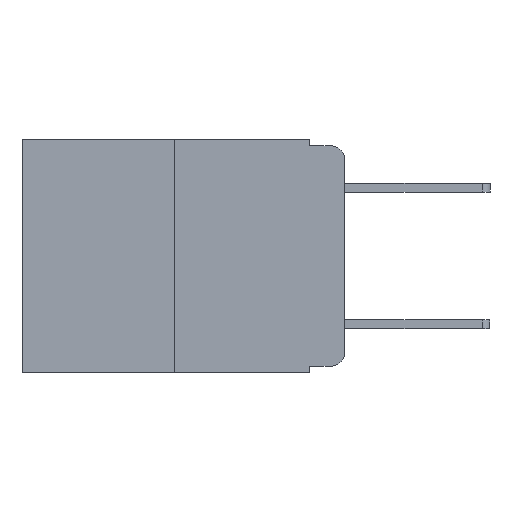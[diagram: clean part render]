
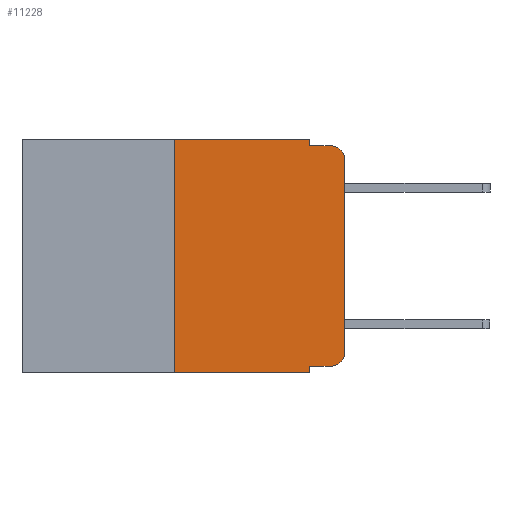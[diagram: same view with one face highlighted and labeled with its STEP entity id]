
A CAD part, left-side view. The second image highlights one B-rep face of the part: STEP entity #11228.
In plain terms, the highlighted planar face has unit normal (-1, 0, 0).
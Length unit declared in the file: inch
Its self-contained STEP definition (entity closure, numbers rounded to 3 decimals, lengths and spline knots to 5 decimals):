
#383 = CARTESIAN_POINT ( 'NONE',  ( 0., 0.25, -0.343 ) ) ;
#790 = CARTESIAN_POINT ( 'NONE',  ( 0., 0.051, -0.01 ) ) ;
#812 = VERTEX_POINT ( 'NONE', #22494 ) ;
#847 = CIRCLE ( 'NONE', #1784, 0.02 ) ;
#1298 = VECTOR ( 'NONE', #4425, 39.37008 ) ;
#1396 = VERTEX_POINT ( 'NONE', #383 ) ;
#1666 = DIRECTION ( 'NONE',  ( 0., -1., 0. ) ) ;
#1784 = AXIS2_PLACEMENT_3D ( 'NONE', #4016, #16246, #5816 ) ;
#2018 = FACE_OUTER_BOUND ( 'NONE', #10277, .T. ) ;
#2053 = VERTEX_POINT ( 'NONE', #8098 ) ;
#2700 = ORIENTED_EDGE ( 'NONE', *, *, #22243, .F. ) ;
#3367 = CARTESIAN_POINT ( 'NONE',  ( 0., 0.02, -0.03 ) ) ;
#3387 = DIRECTION ( 'NONE',  ( -1., 0., 0. ) ) ;
#4016 = CARTESIAN_POINT ( 'NONE',  ( 0., 0.02, -0.313 ) ) ;
#4325 = CARTESIAN_POINT ( 'NONE',  ( 0., 0., -0.03 ) ) ;
#4377 = CARTESIAN_POINT ( 'NONE',  ( 0., 0.051, 0. ) ) ;
#4425 = DIRECTION ( 'NONE',  ( 0., 0., 1. ) ) ;
#4744 = CARTESIAN_POINT ( 'NONE',  ( 0., 0.051, 0. ) ) ;
#4896 = EDGE_CURVE ( 'NONE', #10348, #2053, #16150, .T. ) ;
#4917 = ORIENTED_EDGE ( 'NONE', *, *, #20403, .T. ) ;
#4985 = DIRECTION ( 'NONE',  ( 1., 0., 0. ) ) ;
#5081 = ORIENTED_EDGE ( 'NONE', *, *, #18565, .T. ) ;
#5100 = VECTOR ( 'NONE', #22039, 39.37008 ) ;
#5471 = ORIENTED_EDGE ( 'NONE', *, *, #4896, .T. ) ;
#5792 = DIRECTION ( 'NONE',  ( 0., 0., -1. ) ) ;
#5816 = DIRECTION ( 'NONE',  ( 0., 0., -1. ) ) ;
#5966 = LINE ( 'NONE', #18441, #14667 ) ;
#6220 = LINE ( 'NONE', #13113, #1298 ) ;
#7492 = DIRECTION ( 'NONE',  ( 0., -1., 0. ) ) ;
#8098 = CARTESIAN_POINT ( 'NONE',  ( 0., 0.02, -0.01 ) ) ;
#8841 = LINE ( 'NONE', #10596, #21511 ) ;
#8930 = LINE ( 'NONE', #11008, #17608 ) ;
#9067 = LINE ( 'NONE', #22027, #17215 ) ;
#9083 = VERTEX_POINT ( 'NONE', #12983 ) ;
#10277 = EDGE_LOOP ( 'NONE', ( #4917, #5471, #20347, #12271, #19557, #18804, #20388, #2700, #19143, #5081 ) ) ;
#10348 = VERTEX_POINT ( 'NONE', #4325 ) ;
#10406 = CARTESIAN_POINT ( 'NONE',  ( 0., 0., -0.313 ) ) ;
#10557 = CARTESIAN_POINT ( 'NONE',  ( 0., 0.051, -0.343 ) ) ;
#10596 = CARTESIAN_POINT ( 'NONE',  ( 0., 0.473, -0.343 ) ) ;
#11008 = CARTESIAN_POINT ( 'NONE',  ( 0., 0.473, 0. ) ) ;
#11109 = VERTEX_POINT ( 'NONE', #790 ) ;
#11168 = VECTOR ( 'NONE', #19277, 39.37008 ) ;
#11228 = ADVANCED_FACE ( 'NONE', ( #2018 ), #15443, .F. ) ;
#11394 = LINE ( 'NONE', #4744, #5100 ) ;
#11719 = LINE ( 'NONE', #19201, #11168 ) ;
#12271 = ORIENTED_EDGE ( 'NONE', *, *, #14221, .F. ) ;
#12921 = EDGE_CURVE ( 'NONE', #12965, #19096, #8930, .T. ) ;
#12965 = VERTEX_POINT ( 'NONE', #21450 ) ;
#12983 = CARTESIAN_POINT ( 'NONE',  ( 0., 0.02, -0.333 ) ) ;
#13071 = EDGE_CURVE ( 'NONE', #1396, #12965, #6220, .T. ) ;
#13113 = CARTESIAN_POINT ( 'NONE',  ( 0., 0.25, 0. ) ) ;
#14012 = VECTOR ( 'NONE', #19980, 39.37008 ) ;
#14221 = EDGE_CURVE ( 'NONE', #19096, #11109, #18622, .T. ) ;
#14667 = VECTOR ( 'NONE', #20135, 39.37008 ) ;
#15253 = DIRECTION ( 'NONE',  ( 0., -1., 0. ) ) ;
#15411 = VERTEX_POINT ( 'NONE', #10406 ) ;
#15443 = PLANE ( 'NONE',  #19037 ) ;
#16150 = CIRCLE ( 'NONE', #17678, 0.02 ) ;
#16246 = DIRECTION ( 'NONE',  ( -1., 0., 0. ) ) ;
#17165 = DIRECTION ( 'NONE',  ( 0., 0., -1. ) ) ;
#17215 = VECTOR ( 'NONE', #15253, 39.37008 ) ;
#17608 = VECTOR ( 'NONE', #7492, 39.37008 ) ;
#17678 = AXIS2_PLACEMENT_3D ( 'NONE', #3367, #3387, #5792 ) ;
#17739 = EDGE_CURVE ( 'NONE', #1396, #20649, #8841, .T. ) ;
#18441 = CARTESIAN_POINT ( 'NONE',  ( 0., 0.051, -0.01 ) ) ;
#18565 = EDGE_CURVE ( 'NONE', #9083, #15411, #847, .T. ) ;
#18622 = LINE ( 'NONE', #4377, #14012 ) ;
#18804 = ORIENTED_EDGE ( 'NONE', *, *, #13071, .F. ) ;
#18849 = EDGE_CURVE ( 'NONE', #812, #9083, #9067, .T. ) ;
#19037 = AXIS2_PLACEMENT_3D ( 'NONE', #20501, #4985, #17165 ) ;
#19096 = VERTEX_POINT ( 'NONE', #22656 ) ;
#19143 = ORIENTED_EDGE ( 'NONE', *, *, #18849, .T. ) ;
#19201 = CARTESIAN_POINT ( 'NONE',  ( 0., 0., 0. ) ) ;
#19277 = DIRECTION ( 'NONE',  ( 0., 0., 1. ) ) ;
#19557 = ORIENTED_EDGE ( 'NONE', *, *, #12921, .F. ) ;
#19980 = DIRECTION ( 'NONE',  ( 0., 0., -1. ) ) ;
#20135 = DIRECTION ( 'NONE',  ( 0., -1., 0. ) ) ;
#20347 = ORIENTED_EDGE ( 'NONE', *, *, #21558, .F. ) ;
#20388 = ORIENTED_EDGE ( 'NONE', *, *, #17739, .T. ) ;
#20403 = EDGE_CURVE ( 'NONE', #15411, #10348, #11719, .T. ) ;
#20501 = CARTESIAN_POINT ( 'NONE',  ( 0., 0.473, 0. ) ) ;
#20649 = VERTEX_POINT ( 'NONE', #10557 ) ;
#21450 = CARTESIAN_POINT ( 'NONE',  ( 0., 0.25, 0. ) ) ;
#21511 = VECTOR ( 'NONE', #1666, 39.37008 ) ;
#21558 = EDGE_CURVE ( 'NONE', #11109, #2053, #5966, .T. ) ;
#22027 = CARTESIAN_POINT ( 'NONE',  ( 0., 0.051, -0.333 ) ) ;
#22039 = DIRECTION ( 'NONE',  ( 0., 0., -1. ) ) ;
#22243 = EDGE_CURVE ( 'NONE', #812, #20649, #11394, .T. ) ;
#22494 = CARTESIAN_POINT ( 'NONE',  ( 0., 0.051, -0.333 ) ) ;
#22656 = CARTESIAN_POINT ( 'NONE',  ( 0., 0.051, 0. ) ) ;
